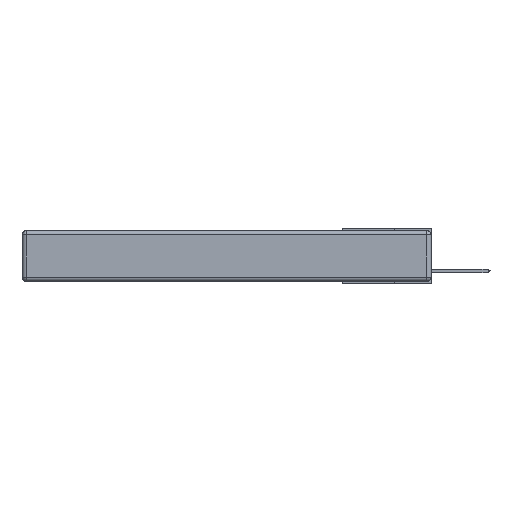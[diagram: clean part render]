
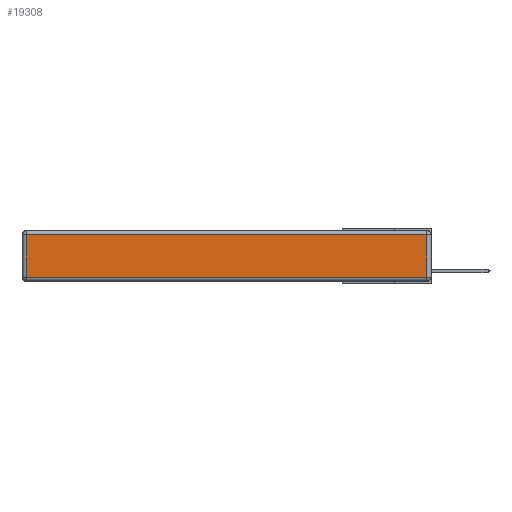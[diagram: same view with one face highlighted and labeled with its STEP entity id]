
A CAD part, left-side view. The second image highlights one B-rep face of the part: STEP entity #19308.
In plain terms, the highlighted planar face has unit normal (-1, 0, 0).
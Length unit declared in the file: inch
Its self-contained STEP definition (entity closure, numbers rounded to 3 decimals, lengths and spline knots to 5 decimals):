
#67 = VERTEX_POINT ( 'NONE', #9942 ) ;
#844 = CARTESIAN_POINT ( 'NONE',  ( 0., 2.72, -0.03 ) ) ;
#1418 = CARTESIAN_POINT ( 'NONE',  ( 0., 0.03, -0.313 ) ) ;
#1439 = FACE_OUTER_BOUND ( 'NONE', #18024, .T. ) ;
#2884 = VERTEX_POINT ( 'NONE', #8712 ) ;
#2896 = ORIENTED_EDGE ( 'NONE', *, *, #5041, .T. ) ;
#3304 = DIRECTION ( 'NONE',  ( 0., 0., -1. ) ) ;
#4044 = EDGE_CURVE ( 'NONE', #14965, #67, #21072, .T. ) ;
#4251 = DIRECTION ( 'NONE',  ( 0., 0., 1. ) ) ;
#5041 = EDGE_CURVE ( 'NONE', #6723, #2884, #8508, .T. ) ;
#5705 = DIRECTION ( 'NONE',  ( -1., 0., 0. ) ) ;
#5845 = CARTESIAN_POINT ( 'NONE',  ( 0., 2.75, -0.03 ) ) ;
#6723 = VERTEX_POINT ( 'NONE', #844 ) ;
#6797 = CARTESIAN_POINT ( 'NONE',  ( 0., 2.72, -0.343 ) ) ;
#8508 = LINE ( 'NONE', #6797, #10731 ) ;
#8712 = CARTESIAN_POINT ( 'NONE',  ( 0., 2.72, -0.313 ) ) ;
#9779 = EDGE_CURVE ( 'NONE', #67, #6723, #17268, .T. ) ;
#9942 = CARTESIAN_POINT ( 'NONE',  ( 0., 0.03, -0.03 ) ) ;
#10631 = CARTESIAN_POINT ( 'NONE',  ( 0., 0., -0.313 ) ) ;
#10731 = VECTOR ( 'NONE', #3304, 39.37008 ) ;
#12340 = DIRECTION ( 'NONE',  ( 0., -1., 0. ) ) ;
#13239 = AXIS2_PLACEMENT_3D ( 'NONE', #16892, #5705, #18661 ) ;
#13627 = EDGE_CURVE ( 'NONE', #2884, #14965, #17592, .T. ) ;
#14866 = CARTESIAN_POINT ( 'NONE',  ( 0., 0.03, -0.343 ) ) ;
#14963 = VECTOR ( 'NONE', #4251, 39.37008 ) ;
#14965 = VERTEX_POINT ( 'NONE', #1418 ) ;
#15073 = VECTOR ( 'NONE', #16930, 39.37008 ) ;
#16088 = ORIENTED_EDGE ( 'NONE', *, *, #4044, .T. ) ;
#16892 = CARTESIAN_POINT ( 'NONE',  ( 0., 0., -0.343 ) ) ;
#16893 = ORIENTED_EDGE ( 'NONE', *, *, #13627, .T. ) ;
#16930 = DIRECTION ( 'NONE',  ( 0., 1., 0. ) ) ;
#17268 = LINE ( 'NONE', #5845, #15073 ) ;
#17592 = LINE ( 'NONE', #10631, #19560 ) ;
#18024 = EDGE_LOOP ( 'NONE', ( #16893, #16088, #20108, #2896 ) ) ;
#18661 = DIRECTION ( 'NONE',  ( 0., 0., 1. ) ) ;
#19308 = ADVANCED_FACE ( 'NONE', ( #1439 ), #20648, .T. ) ;
#19560 = VECTOR ( 'NONE', #12340, 39.37008 ) ;
#20108 = ORIENTED_EDGE ( 'NONE', *, *, #9779, .T. ) ;
#20648 = PLANE ( 'NONE',  #13239 ) ;
#21072 = LINE ( 'NONE', #14866, #14963 ) ;
